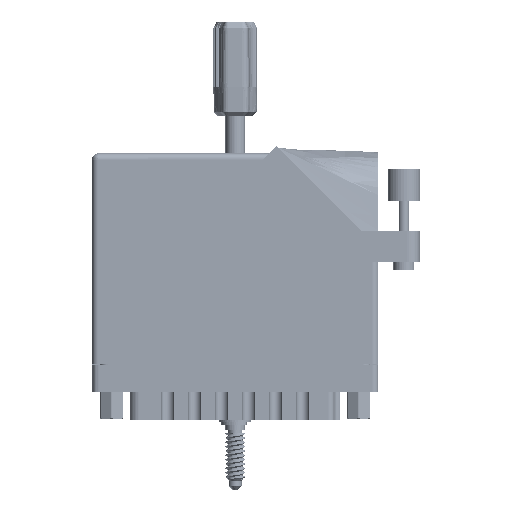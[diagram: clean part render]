
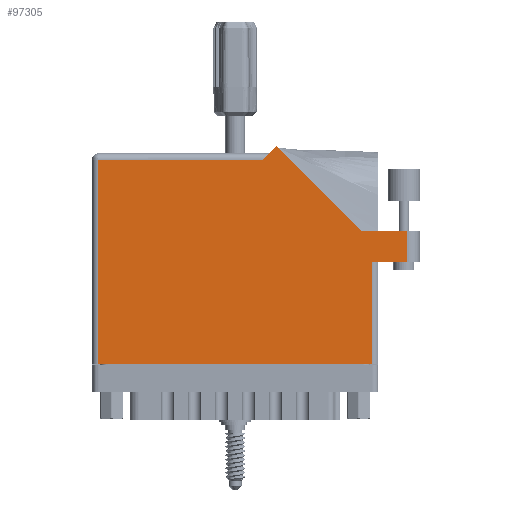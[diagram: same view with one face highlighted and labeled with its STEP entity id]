
A CAD part, front view. The second image highlights one B-rep face of the part: STEP entity #97305.
In plain terms, the highlighted face is planar.
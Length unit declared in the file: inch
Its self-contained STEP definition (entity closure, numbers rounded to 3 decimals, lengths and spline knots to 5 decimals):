
#1236 = CARTESIAN_POINT ( 'NONE',  ( 2.693, 0.98, 0. ) ) ;
#1256 = VERTEX_POINT ( 'NONE', #109719 ) ;
#2020 = ORIENTED_EDGE ( 'NONE', *, *, #78209, .T. ) ;
#2333 = VERTEX_POINT ( 'NONE', #71134 ) ;
#3003 = EDGE_CURVE ( 'NONE', #1256, #10945, #112907, .T. ) ;
#3633 = VERTEX_POINT ( 'NONE', #110367 ) ;
#4350 = FACE_OUTER_BOUND ( 'NONE', #63428, .T. ) ;
#6214 = VECTOR ( 'NONE', #27367, 39.37008 ) ;
#8906 = ORIENTED_EDGE ( 'NONE', *, *, #29278, .T. ) ;
#10945 = VERTEX_POINT ( 'NONE', #74951 ) ;
#11552 = AXIS2_PLACEMENT_3D ( 'NONE', #75905, #93983, #28592 ) ;
#11651 = EDGE_CURVE ( 'NONE', #60460, #1256, #52755, .T. ) ;
#14119 = DIRECTION ( 'NONE',  ( -1., 0., 0. ) ) ;
#15210 = VECTOR ( 'NONE', #109873, 39.37008 ) ;
#16499 = CARTESIAN_POINT ( 'NONE',  ( 3.155, 1.287, 0. ) ) ;
#16847 = LINE ( 'NONE', #39137, #25442 ) ;
#18247 = CARTESIAN_POINT ( 'NONE',  ( 0., 0., 0. ) ) ;
#18358 = LINE ( 'NONE', #16499, #88794 ) ;
#21082 = CARTESIAN_POINT ( 'NONE',  ( 2.693, 0.98, 0. ) ) ;
#23344 = ORIENTED_EDGE ( 'NONE', *, *, #54741, .T. ) ;
#24342 = VECTOR ( 'NONE', #14119, 39.37008 ) ;
#25442 = VECTOR ( 'NONE', #56366, 39.37008 ) ;
#27367 = DIRECTION ( 'NONE',  ( 1., 0., 0. ) ) ;
#27830 = CARTESIAN_POINT ( 'NONE',  ( 1.705, 2.03, 0. ) ) ;
#28592 = DIRECTION ( 'NONE',  ( -1., 0., 0. ) ) ;
#29278 = EDGE_CURVE ( 'NONE', #94985, #30798, #30744, .T. ) ;
#29599 = ORIENTED_EDGE ( 'NONE', *, *, #11651, .T. ) ;
#30744 = LINE ( 'NONE', #82352, #6214 ) ;
#30798 = VERTEX_POINT ( 'NONE', #92243 ) ;
#31250 = VECTOR ( 'NONE', #48251, 39.37008 ) ;
#38907 = LINE ( 'NONE', #1236, #84798 ) ;
#39137 = CARTESIAN_POINT ( 'NONE',  ( 0.062, 0., 0. ) ) ;
#40992 = EDGE_CURVE ( 'NONE', #3633, #94985, #38907, .T. ) ;
#45450 = DIRECTION ( 'NONE',  ( -1., 0., 0. ) ) ;
#47377 = VERTEX_POINT ( 'NONE', #73071 ) ;
#48170 = PLANE ( 'NONE',  #11552 ) ;
#48251 = DIRECTION ( 'NONE',  ( -0.707, 0.707, 0. ) ) ;
#49622 = DIRECTION ( 'NONE',  ( 0., 1., 0. ) ) ;
#52755 = LINE ( 'NONE', #85948, #31250 ) ;
#53996 = ORIENTED_EDGE ( 'NONE', *, *, #64296, .T. ) ;
#54741 = EDGE_CURVE ( 'NONE', #10945, #47377, #97676, .T. ) ;
#56366 = DIRECTION ( 'NONE',  ( 0., -1., 0. ) ) ;
#59948 = CARTESIAN_POINT ( 'NONE',  ( 0., 1.968, 0. ) ) ;
#60460 = VERTEX_POINT ( 'NONE', #118520 ) ;
#63428 = EDGE_LOOP ( 'NONE', ( #8906, #53996, #116996, #29599, #81901, #23344, #2020, #99423, #88539 ) ) ;
#64296 = EDGE_CURVE ( 'NONE', #30798, #77736, #101772, .T. ) ;
#71134 = CARTESIAN_POINT ( 'NONE',  ( 0.062, 0., 0. ) ) ;
#73071 = CARTESIAN_POINT ( 'NONE',  ( 0.062, 1.968, 0. ) ) ;
#74951 = CARTESIAN_POINT ( 'NONE',  ( 1.643, 1.968, 0. ) ) ;
#75905 = CARTESIAN_POINT ( 'NONE',  ( 0., 2.03, 0. ) ) ;
#77736 = VERTEX_POINT ( 'NONE', #115841 ) ;
#78209 = EDGE_CURVE ( 'NONE', #47377, #2333, #16847, .T. ) ;
#78541 = EDGE_CURVE ( 'NONE', #77736, #60460, #18358, .T. ) ;
#81901 = ORIENTED_EDGE ( 'NONE', *, *, #3003, .T. ) ;
#82352 = CARTESIAN_POINT ( 'NONE',  ( 2.755, 0.98, 0. ) ) ;
#83607 = VECTOR ( 'NONE', #91777, 39.37008 ) ;
#84798 = VECTOR ( 'NONE', #92475, 39.37008 ) ;
#85948 = CARTESIAN_POINT ( 'NONE',  ( 2.58942, 1.287, 0. ) ) ;
#86127 = CARTESIAN_POINT ( 'NONE',  ( 3.03, 1.287, 0. ) ) ;
#88539 = ORIENTED_EDGE ( 'NONE', *, *, #40992, .T. ) ;
#88794 = VECTOR ( 'NONE', #45450, 39.37008 ) ;
#91777 = DIRECTION ( 'NONE',  ( 1., 0., 0. ) ) ;
#92243 = CARTESIAN_POINT ( 'NONE',  ( 3.03, 0.98, 0. ) ) ;
#92475 = DIRECTION ( 'NONE',  ( 0., 1., 0. ) ) ;
#93983 = DIRECTION ( 'NONE',  ( 0., 0., -1. ) ) ;
#94985 = VERTEX_POINT ( 'NONE', #21082 ) ;
#97305 = ADVANCED_FACE ( 'NONE', ( #4350 ), #48170, .F. ) ;
#97676 = LINE ( 'NONE', #59948, #24342 ) ;
#99423 = ORIENTED_EDGE ( 'NONE', *, *, #112937, .T. ) ;
#101772 = LINE ( 'NONE', #86127, #103144 ) ;
#102320 = LINE ( 'NONE', #18247, #83607 ) ;
#103144 = VECTOR ( 'NONE', #49622, 39.37008 ) ;
#109719 = CARTESIAN_POINT ( 'NONE',  ( 1.77571, 2.10071, 0. ) ) ;
#109873 = DIRECTION ( 'NONE',  ( -0.707, -0.707, 0. ) ) ;
#110367 = CARTESIAN_POINT ( 'NONE',  ( 2.693, 0., 0. ) ) ;
#112907 = LINE ( 'NONE', #27830, #15210 ) ;
#112937 = EDGE_CURVE ( 'NONE', #2333, #3633, #102320, .T. ) ;
#115841 = CARTESIAN_POINT ( 'NONE',  ( 3.03, 1.287, 0. ) ) ;
#116996 = ORIENTED_EDGE ( 'NONE', *, *, #78541, .T. ) ;
#118520 = CARTESIAN_POINT ( 'NONE',  ( 2.58942, 1.287, 0. ) ) ;
